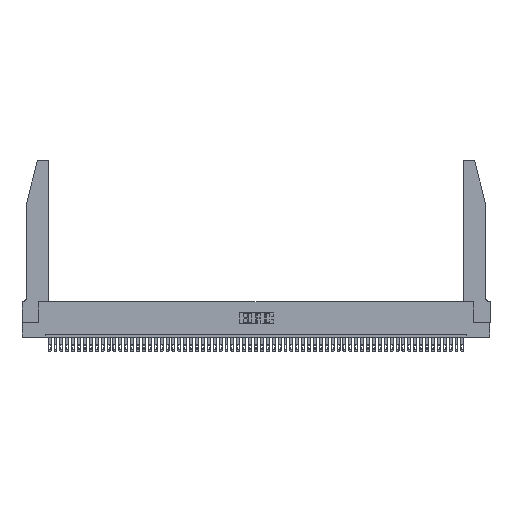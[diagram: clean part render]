
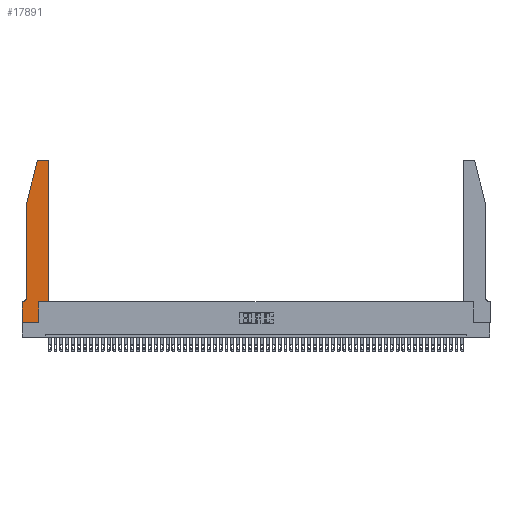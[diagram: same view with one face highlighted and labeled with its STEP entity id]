
A CAD part, top view. The second image highlights one B-rep face of the part: STEP entity #17891.
In plain terms, the highlighted planar face has unit normal (0, 0, 1).
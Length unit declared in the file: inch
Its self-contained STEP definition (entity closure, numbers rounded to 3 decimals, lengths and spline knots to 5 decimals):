
#304 = CARTESIAN_POINT ( 'NONE',  ( 0.4505, 0.35, 0.37 ) ) ;
#397 = DIRECTION ( 'NONE',  ( 0., -1., 0. ) ) ;
#616 = VECTOR ( 'NONE', #41402, 39.37008 ) ;
#715 = DIRECTION ( 'NONE',  ( 1., 0., 0. ) ) ;
#974 = DIRECTION ( 'NONE',  ( 0., 0., -1. ) ) ;
#1184 = DIRECTION ( 'NONE',  ( 0., 1., 0. ) ) ;
#1383 = VECTOR ( 'NONE', #39290, 39.37008 ) ;
#1809 = VERTEX_POINT ( 'NONE', #26136 ) ;
#2528 = ORIENTED_EDGE ( 'NONE', *, *, #52668, .T. ) ;
#3131 = ORIENTED_EDGE ( 'NONE', *, *, #45951, .T. ) ;
#3168 = CARTESIAN_POINT ( 'NONE',  ( 0.4205, 2.72, 0.37 ) ) ;
#3614 = EDGE_CURVE ( 'NONE', #47233, #23995, #49513, .T. ) ;
#3748 = ORIENTED_EDGE ( 'NONE', *, *, #28662, .T. ) ;
#4435 = EDGE_LOOP ( 'NONE', ( #3748, #15085, #23204, #3131, #48954, #8877, #18203, #31472, #54055, #2528, #38439, #26945 ) ) ;
#5354 = LINE ( 'NONE', #20376, #34878 ) ;
#5469 = VECTOR ( 'NONE', #28027, 39.37008 ) ;
#7509 = VERTEX_POINT ( 'NONE', #31896 ) ;
#7678 = EDGE_CURVE ( 'NONE', #13185, #42551, #53292, .T. ) ;
#8010 = VERTEX_POINT ( 'NONE', #44399 ) ;
#8336 = DIRECTION ( 'NONE',  ( 1., 0., 0. ) ) ;
#8677 = CARTESIAN_POINT ( 'NONE',  ( 0., 0.35, 0.37 ) ) ;
#8744 = CARTESIAN_POINT ( 'NONE',  ( 0.0755, 2., 0.37 ) ) ;
#8877 = ORIENTED_EDGE ( 'NONE', *, *, #49319, .T. ) ;
#8972 = CARTESIAN_POINT ( 'NONE',  ( 0.25487, 2.72718, 0.37 ) ) ;
#10353 = VERTEX_POINT ( 'NONE', #10987 ) ;
#10967 = PLANE ( 'NONE',  #48690 ) ;
#10987 = CARTESIAN_POINT ( 'NONE',  ( 0.0055, 0.35, 0.37 ) ) ;
#12536 = CIRCLE ( 'NONE', #30090, 0.03 ) ;
#12721 = LINE ( 'NONE', #43310, #1383 ) ;
#13185 = VERTEX_POINT ( 'NONE', #19725 ) ;
#13468 = LINE ( 'NONE', #304, #21365 ) ;
#14480 = LINE ( 'NONE', #41214, #616 ) ;
#14545 = LINE ( 'NONE', #24899, #52498 ) ;
#15085 = ORIENTED_EDGE ( 'NONE', *, *, #7678, .T. ) ;
#15183 = CARTESIAN_POINT ( 'NONE',  ( 0., 0.35, 0.37 ) ) ;
#16052 = DIRECTION ( 'NONE',  ( 0., 0., 1. ) ) ;
#16216 = CARTESIAN_POINT ( 'NONE',  ( 0.0755, 0.35, 0.37 ) ) ;
#17001 = CARTESIAN_POINT ( 'NONE',  ( 0.4505, 0.35, 0.37 ) ) ;
#17282 = EDGE_CURVE ( 'NONE', #23995, #31778, #12536, .T. ) ;
#17891 = ADVANCED_FACE ( 'NONE', ( #18938 ), #10967, .T. ) ;
#18203 = ORIENTED_EDGE ( 'NONE', *, *, #45804, .T. ) ;
#18938 = FACE_OUTER_BOUND ( 'NONE', #4435, .T. ) ;
#19400 = VECTOR ( 'NONE', #1184, 39.37008 ) ;
#19725 = CARTESIAN_POINT ( 'NONE',  ( 0.284, 2.75, 0.37 ) ) ;
#19963 = VECTOR ( 'NONE', #50293, 39.37008 ) ;
#20376 = CARTESIAN_POINT ( 'NONE',  ( 0.2605, 2.75, 0.37 ) ) ;
#21365 = VECTOR ( 'NONE', #715, 39.37008 ) ;
#23204 = ORIENTED_EDGE ( 'NONE', *, *, #33933, .T. ) ;
#23995 = VERTEX_POINT ( 'NONE', #33052 ) ;
#24899 = CARTESIAN_POINT ( 'NONE',  ( 0.0755, 2., 0.37 ) ) ;
#24995 = EDGE_CURVE ( 'NONE', #8010, #1809, #42942, .T. ) ;
#25027 = CARTESIAN_POINT ( 'NONE',  ( 0.284, 2.72, 0.37 ) ) ;
#25268 = AXIS2_PLACEMENT_3D ( 'NONE', #30987, #974, #39202 ) ;
#26136 = CARTESIAN_POINT ( 'NONE',  ( 0.2865, 0.35, 0.37 ) ) ;
#26626 = DIRECTION ( 'NONE',  ( -1., 0., 0. ) ) ;
#26945 = ORIENTED_EDGE ( 'NONE', *, *, #17282, .T. ) ;
#28027 = DIRECTION ( 'NONE',  ( 0., 1., 0. ) ) ;
#28305 = DIRECTION ( 'NONE',  ( 1., 0., 0. ) ) ;
#28541 = EDGE_CURVE ( 'NONE', #29169, #8010, #12721, .T. ) ;
#28559 = CARTESIAN_POINT ( 'NONE',  ( 0.4205, 2.75, 0.37 ) ) ;
#28662 = EDGE_CURVE ( 'NONE', #31778, #13185, #5354, .T. ) ;
#29169 = VERTEX_POINT ( 'NONE', #31747 ) ;
#30090 = AXIS2_PLACEMENT_3D ( 'NONE', #3168, #52919, #28305 ) ;
#30987 = CARTESIAN_POINT ( 'NONE',  ( 0.0055, 0.42, 0.37 ) ) ;
#31472 = ORIENTED_EDGE ( 'NONE', *, *, #28541, .T. ) ;
#31747 = CARTESIAN_POINT ( 'NONE',  ( 0., 0., 0.37 ) ) ;
#31778 = VERTEX_POINT ( 'NONE', #28559 ) ;
#31896 = CARTESIAN_POINT ( 'NONE',  ( 0.0755, 2., 0.37 ) ) ;
#32119 = VERTEX_POINT ( 'NONE', #48911 ) ;
#33052 = CARTESIAN_POINT ( 'NONE',  ( 0.4505, 2.72, 0.37 ) ) ;
#33933 = EDGE_CURVE ( 'NONE', #42551, #7509, #39528, .T. ) ;
#34878 = VECTOR ( 'NONE', #26626, 39.37008 ) ;
#35754 = LINE ( 'NONE', #16216, #50775 ) ;
#35817 = CIRCLE ( 'NONE', #25268, 0.07 ) ;
#38439 = ORIENTED_EDGE ( 'NONE', *, *, #3614, .T. ) ;
#39202 = DIRECTION ( 'NONE',  ( -1., 0., 0. ) ) ;
#39290 = DIRECTION ( 'NONE',  ( 1., 0., 0. ) ) ;
#39502 = DIRECTION ( 'NONE',  ( 1., 0., 0. ) ) ;
#39528 = LINE ( 'NONE', #8744, #19963 ) ;
#40869 = VERTEX_POINT ( 'NONE', #8677 ) ;
#41214 = CARTESIAN_POINT ( 'NONE',  ( 0., 0., 0.37 ) ) ;
#41402 = DIRECTION ( 'NONE',  ( 0., -1., 0. ) ) ;
#42110 = EDGE_CURVE ( 'NONE', #32119, #10353, #35817, .T. ) ;
#42551 = VERTEX_POINT ( 'NONE', #8972 ) ;
#42942 = LINE ( 'NONE', #53756, #19400 ) ;
#43310 = CARTESIAN_POINT ( 'NONE',  ( 0., 0., 0.37 ) ) ;
#44399 = CARTESIAN_POINT ( 'NONE',  ( 0.2865, 0., 0.37 ) ) ;
#44682 = CARTESIAN_POINT ( 'NONE',  ( 0.4505, 0.35, 0.37 ) ) ;
#45804 = EDGE_CURVE ( 'NONE', #40869, #29169, #14480, .T. ) ;
#45951 = EDGE_CURVE ( 'NONE', #7509, #32119, #14545, .T. ) ;
#47233 = VERTEX_POINT ( 'NONE', #17001 ) ;
#48690 = AXIS2_PLACEMENT_3D ( 'NONE', #15183, #52234, #39502 ) ;
#48911 = CARTESIAN_POINT ( 'NONE',  ( 0.0755, 0.42, 0.37 ) ) ;
#48954 = ORIENTED_EDGE ( 'NONE', *, *, #42110, .T. ) ;
#49319 = EDGE_CURVE ( 'NONE', #10353, #40869, #35754, .T. ) ;
#49513 = LINE ( 'NONE', #44682, #5469 ) ;
#50293 = DIRECTION ( 'NONE',  ( -0.239, -0.971, 0. ) ) ;
#50775 = VECTOR ( 'NONE', #53309, 39.37008 ) ;
#52234 = DIRECTION ( 'NONE',  ( 0., 0., 1. ) ) ;
#52498 = VECTOR ( 'NONE', #397, 39.37008 ) ;
#52668 = EDGE_CURVE ( 'NONE', #1809, #47233, #13468, .T. ) ;
#52919 = DIRECTION ( 'NONE',  ( 0., 0., 1. ) ) ;
#53292 = CIRCLE ( 'NONE', #53933, 0.03 ) ;
#53309 = DIRECTION ( 'NONE',  ( -1., 0., 0. ) ) ;
#53756 = CARTESIAN_POINT ( 'NONE',  ( 0.2865, 0.35, 0.37 ) ) ;
#53933 = AXIS2_PLACEMENT_3D ( 'NONE', #25027, #16052, #8336 ) ;
#54055 = ORIENTED_EDGE ( 'NONE', *, *, #24995, .T. ) ;
